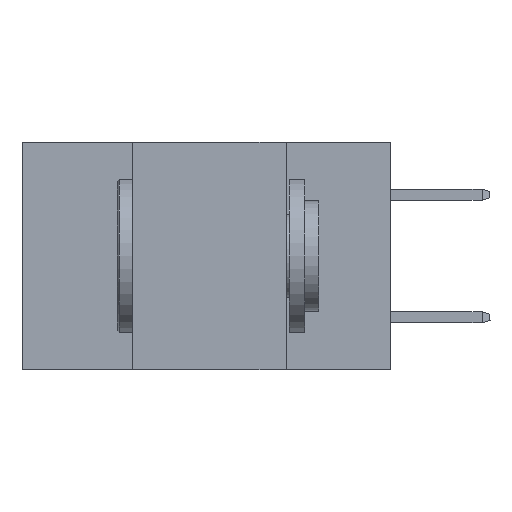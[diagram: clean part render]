
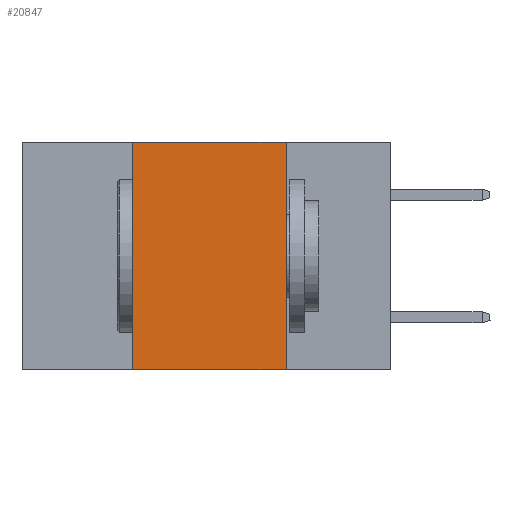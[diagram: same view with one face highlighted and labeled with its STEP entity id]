
A CAD part, left-side view. The second image highlights one B-rep face of the part: STEP entity #20847.
In plain terms, the highlighted planar face has unit normal (-1, 0, 0).
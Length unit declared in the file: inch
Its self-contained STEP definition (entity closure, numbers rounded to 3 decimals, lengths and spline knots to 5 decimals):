
#428 = CARTESIAN_POINT ( 'NONE',  ( 0., 0.17, -0.37 ) ) ;
#1526 = PLANE ( 'NONE',  #3597 ) ;
#1621 = EDGE_CURVE ( 'NONE', #10526, #14869, #12814, .T. ) ;
#3069 = CARTESIAN_POINT ( 'NONE',  ( 0., 0.17, 0. ) ) ;
#3198 = CARTESIAN_POINT ( 'NONE',  ( 0., 0.6, -0.37 ) ) ;
#3597 = AXIS2_PLACEMENT_3D ( 'NONE', #3862, #13273, #15594 ) ;
#3862 = CARTESIAN_POINT ( 'NONE',  ( 0., 0.6, 0. ) ) ;
#4463 = CARTESIAN_POINT ( 'NONE',  ( 0., 0.42, -0.37 ) ) ;
#5570 = VERTEX_POINT ( 'NONE', #428 ) ;
#5778 = ORIENTED_EDGE ( 'NONE', *, *, #8642, .F. ) ;
#7257 = LINE ( 'NONE', #3069, #17373 ) ;
#7383 = VECTOR ( 'NONE', #21026, 39.37008 ) ;
#8554 = FACE_OUTER_BOUND ( 'NONE', #16943, .T. ) ;
#8642 = EDGE_CURVE ( 'NONE', #14869, #5570, #7257, .T. ) ;
#10526 = VERTEX_POINT ( 'NONE', #23555 ) ;
#11305 = ORIENTED_EDGE ( 'NONE', *, *, #25842, .T. ) ;
#11496 = LINE ( 'NONE', #3198, #16573 ) ;
#11937 = CARTESIAN_POINT ( 'NONE',  ( 0., 0.6, 0. ) ) ;
#12814 = LINE ( 'NONE', #11937, #7383 ) ;
#13273 = DIRECTION ( 'NONE',  ( 1., 0., 0. ) ) ;
#14432 = VECTOR ( 'NONE', #25917, 39.37008 ) ;
#14869 = VERTEX_POINT ( 'NONE', #25413 ) ;
#15142 = DIRECTION ( 'NONE',  ( 0., -1., 0. ) ) ;
#15594 = DIRECTION ( 'NONE',  ( 0., 0., -1. ) ) ;
#16565 = ORIENTED_EDGE ( 'NONE', *, *, #1621, .F. ) ;
#16573 = VECTOR ( 'NONE', #15142, 39.37008 ) ;
#16943 = EDGE_LOOP ( 'NONE', ( #5778, #16565, #20747, #11305 ) ) ;
#17373 = VECTOR ( 'NONE', #21571, 39.37008 ) ;
#18707 = EDGE_CURVE ( 'NONE', #24981, #10526, #29923, .T. ) ;
#20747 = ORIENTED_EDGE ( 'NONE', *, *, #18707, .F. ) ;
#20847 = ADVANCED_FACE ( 'NONE', ( #8554 ), #1526, .F. ) ;
#21026 = DIRECTION ( 'NONE',  ( 0., -1., 0. ) ) ;
#21571 = DIRECTION ( 'NONE',  ( 0., 0., -1. ) ) ;
#23555 = CARTESIAN_POINT ( 'NONE',  ( 0., 0.42, 0. ) ) ;
#24981 = VERTEX_POINT ( 'NONE', #4463 ) ;
#25413 = CARTESIAN_POINT ( 'NONE',  ( 0., 0.17, 0. ) ) ;
#25842 = EDGE_CURVE ( 'NONE', #24981, #5570, #11496, .T. ) ;
#25917 = DIRECTION ( 'NONE',  ( 0., 0., 1. ) ) ;
#28040 = CARTESIAN_POINT ( 'NONE',  ( 0., 0.42, 0. ) ) ;
#29923 = LINE ( 'NONE', #28040, #14432 ) ;
